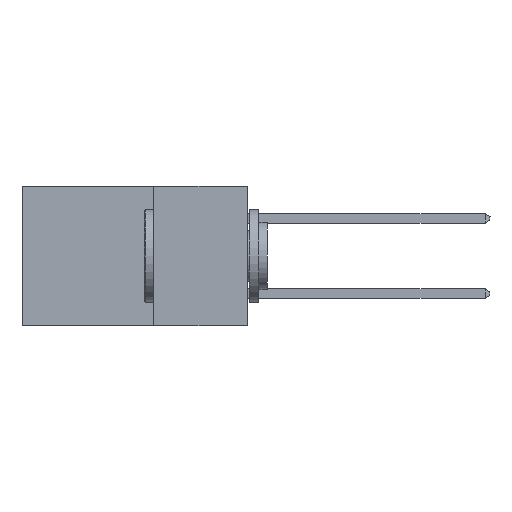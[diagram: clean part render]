
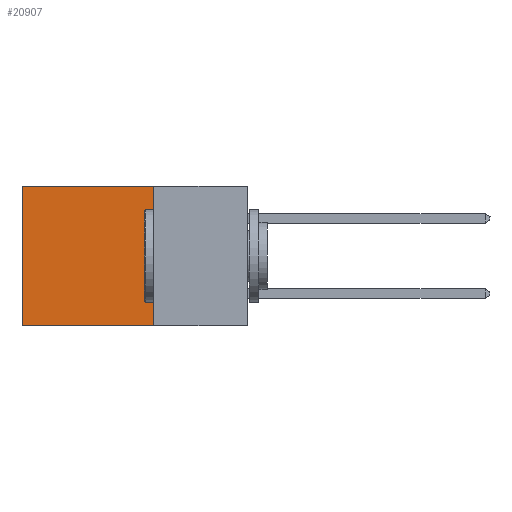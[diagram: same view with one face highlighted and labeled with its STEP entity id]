
A CAD part, left-side view. The second image highlights one B-rep face of the part: STEP entity #20907.
In plain terms, the highlighted planar face has unit normal (-1, 0, 0).
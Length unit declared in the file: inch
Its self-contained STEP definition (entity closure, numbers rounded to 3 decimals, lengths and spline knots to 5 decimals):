
#832 = CARTESIAN_POINT ( 'NONE',  ( 0.298, 0.25, 0. ) ) ;
#1231 = EDGE_CURVE ( 'NONE', #21732, #22717, #13734, .T. ) ;
#4093 = ORIENTED_EDGE ( 'NONE', *, *, #15580, .T. ) ;
#4564 = LINE ( 'NONE', #6303, #16178 ) ;
#4654 = DIRECTION ( 'NONE',  ( 0., 1., 0. ) ) ;
#5519 = CARTESIAN_POINT ( 'NONE',  ( 0.298, 0.25, -0.37 ) ) ;
#6303 = CARTESIAN_POINT ( 'NONE',  ( 0.298, 0.25, 0. ) ) ;
#6925 = VECTOR ( 'NONE', #21126, 39.37008 ) ;
#8857 = DIRECTION ( 'NONE',  ( 0., 0., -1. ) ) ;
#9800 = EDGE_CURVE ( 'NONE', #27037, #21732, #4564, .T. ) ;
#10359 = VERTEX_POINT ( 'NONE', #33022 ) ;
#11024 = CARTESIAN_POINT ( 'NONE',  ( 0.298, 0.25, 0. ) ) ;
#13734 = LINE ( 'NONE', #5519, #6925 ) ;
#14756 = ORIENTED_EDGE ( 'NONE', *, *, #32696, .T. ) ;
#15580 = EDGE_CURVE ( 'NONE', #10359, #22717, #21889, .T. ) ;
#16178 = VECTOR ( 'NONE', #24271, 39.37008 ) ;
#16689 = VECTOR ( 'NONE', #4654, 39.37008 ) ;
#17781 = CARTESIAN_POINT ( 'NONE',  ( 0.298, 0.25, -0.37 ) ) ;
#18014 = FACE_OUTER_BOUND ( 'NONE', #22476, .T. ) ;
#18789 = DIRECTION ( 'NONE',  ( 1., 0., 0. ) ) ;
#20907 = ADVANCED_FACE ( 'NONE', ( #18014 ), #29045, .F. ) ;
#21126 = DIRECTION ( 'NONE',  ( 0., 1., 0. ) ) ;
#21364 = DIRECTION ( 'NONE',  ( 0., 0., -1. ) ) ;
#21421 = CARTESIAN_POINT ( 'NONE',  ( 0.298, 0.6, 0. ) ) ;
#21732 = VERTEX_POINT ( 'NONE', #17781 ) ;
#21889 = LINE ( 'NONE', #21421, #32359 ) ;
#22476 = EDGE_LOOP ( 'NONE', ( #4093, #30446, #26819, #14756 ) ) ;
#22717 = VERTEX_POINT ( 'NONE', #27295 ) ;
#24271 = DIRECTION ( 'NONE',  ( 0., 0., -1. ) ) ;
#26819 = ORIENTED_EDGE ( 'NONE', *, *, #9800, .F. ) ;
#27037 = VERTEX_POINT ( 'NONE', #11024 ) ;
#27295 = CARTESIAN_POINT ( 'NONE',  ( 0.298, 0.6, -0.37 ) ) ;
#28385 = LINE ( 'NONE', #29599, #16689 ) ;
#29045 = PLANE ( 'NONE',  #30956 ) ;
#29599 = CARTESIAN_POINT ( 'NONE',  ( 0.298, 0.25, 0. ) ) ;
#30446 = ORIENTED_EDGE ( 'NONE', *, *, #1231, .F. ) ;
#30956 = AXIS2_PLACEMENT_3D ( 'NONE', #832, #18789, #21364 ) ;
#32359 = VECTOR ( 'NONE', #8857, 39.37008 ) ;
#32696 = EDGE_CURVE ( 'NONE', #27037, #10359, #28385, .T. ) ;
#33022 = CARTESIAN_POINT ( 'NONE',  ( 0.298, 0.6, 0. ) ) ;
